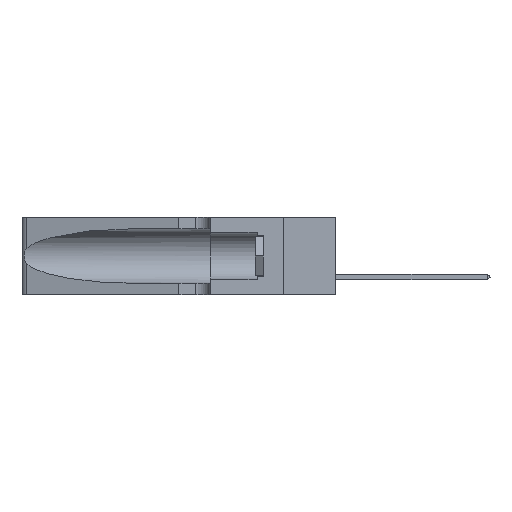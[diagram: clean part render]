
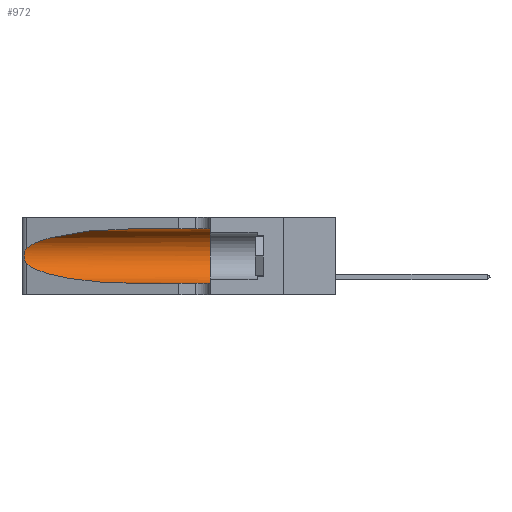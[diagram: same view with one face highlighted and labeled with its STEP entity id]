
A CAD part, left-side view. The second image highlights one B-rep face of the part: STEP entity #972.
In plain terms, the highlighted cylindrical face has radius 3.308 mm (diameter 6.617 mm), a partial arc.
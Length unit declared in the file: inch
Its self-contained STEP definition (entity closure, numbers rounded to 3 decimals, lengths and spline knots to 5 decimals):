
#449 = CARTESIAN_POINT ( 'NONE',  ( 0.25487, 1.22718, 0.14631 ) ) ;
#681 = AXIS2_PLACEMENT_3D ( 'NONE', #48980, #38455, #11279 ) ;
#937 = CARTESIAN_POINT ( 'NONE',  ( 0.25487, 1.22718, 0.22369 ) ) ;
#972 = ADVANCED_FACE ( 'NONE', ( #47488 ), #1754, .F. ) ;
#1268 = ORIENTED_EDGE ( 'NONE', *, *, #25857, .F. ) ;
#1339 = CARTESIAN_POINT ( 'NONE',  ( 0.1305, 1.61858, 0.185 ) ) ;
#1754 = CYLINDRICAL_SURFACE ( 'NONE', #24909, 0.13025 ) ;
#3576 = CARTESIAN_POINT ( 'NONE',  ( 0.2373, 1.15595, 0.08982 ) ) ;
#4775 = CARTESIAN_POINT ( 'NONE',  ( 0.1305, 0.35, 0.05475 ) ) ;
#6134 = CARTESIAN_POINT ( 'NONE',  ( 0.25555, 1.22994, 0.2215 ) ) ;
#6475 = CARTESIAN_POINT ( 'NONE',  ( 0.25787, 1.23484, 0.2124 ) ) ;
#8892 = CARTESIAN_POINT ( 'NONE',  ( 0.1305, 0.72297, 0.05475 ) ) ;
#11030 = CARTESIAN_POINT ( 'NONE',  ( 0.26017, 1.23833, 0.17102 ) ) ;
#11052 = ORIENTED_EDGE ( 'NONE', *, *, #31188, .F. ) ;
#11162 = EDGE_CURVE ( 'NONE', #36340, #18987, #49868, .T. ) ;
#11279 = DIRECTION ( 'NONE',  ( 0., 0., 1. ) ) ;
#11449 = ORIENTED_EDGE ( 'NONE', *, *, #23421, .T. ) ;
#12258 = CARTESIAN_POINT ( 'NONE',  ( 0.25555, 1.22993, 0.14849 ) ) ;
#12418 = CARTESIAN_POINT ( 'NONE',  ( 0.1305, 1.61858, 0.05475 ) ) ;
#14858 = CARTESIAN_POINT ( 'NONE',  ( 0.1305, 0.35, 0.31525 ) ) ;
#15594 = LINE ( 'NONE', #12418, #34826 ) ;
#16298 = DIRECTION ( 'NONE',  ( 0., -1., 0. ) ) ;
#17581 = ORIENTED_EDGE ( 'NONE', *, *, #11162, .T. ) ;
#18987 = VERTEX_POINT ( 'NONE', #34523 ) ;
#19622 = CARTESIAN_POINT ( 'NONE',  ( 0.1305, 0.72297, 0.31525 ) ) ;
#19818 = DIRECTION ( 'NONE',  ( 0., 0., -1. ) ) ;
#20849 = EDGE_CURVE ( 'NONE', #45648, #36340, #28413, .T. ) ;
#20927 = VERTEX_POINT ( 'NONE', #4775 ) ;
#22044 = VERTEX_POINT ( 'NONE', #14858 ) ;
#23013 = CARTESIAN_POINT ( 'NONE',  ( 0.25639, 1.23186, 0.15144 ) ) ;
#23421 = EDGE_CURVE ( 'NONE', #18987, #20927, #15594, .T. ) ;
#24909 = AXIS2_PLACEMENT_3D ( 'NONE', #1339, #16298, #19818 ) ;
#25857 = EDGE_CURVE ( 'NONE', #41160, #22044, #27773, .T. ) ;
#25876 = CARTESIAN_POINT ( 'NONE',  ( 0.25487, 1.22718, 0.14631 ) ) ;
#26415 = CARTESIAN_POINT ( 'NONE',  ( 0.25789, 1.23486, 0.15765 ) ) ;
#27773 = LINE ( 'NONE', #43423, #40519 ) ;
#28056 = DIRECTION ( 'NONE',  ( 0., -1., 0. ) ) ;
#28413 = B_SPLINE_CURVE_WITH_KNOTS ( 'NONE', 3,
 ( #44272, #6134, #45478, #6475, #45305, #33151, #38370, #46120, #11030, #37879, #26415, #23013, #12258, #449 ),
 .UNSPECIFIED., .F., .F.,
 ( 4, 2, 2, 2, 2, 2, 4 ),
 ( 0., 0.00027, 0.00053, 0.00107, 0.0016, 0.00187, 0.00214 ),
 .UNSPECIFIED. ) ;
#29901 = CARTESIAN_POINT ( 'NONE',  ( 0.1305, 0.72297, 0.31525 ) ) ;
#30822 = CIRCLE ( 'NONE', #681, 0.13025 ) ;
#31183 = CARTESIAN_POINT ( 'NONE',  ( 0.18966, 0.96281, 0.31525 ) ) ;
#31188 = EDGE_CURVE ( 'NONE', #22044, #20927, #30822, .T. ) ;
#33151 = CARTESIAN_POINT ( 'NONE',  ( 0.26018, 1.23835, 0.19895 ) ) ;
#34523 = CARTESIAN_POINT ( 'NONE',  ( 0.1305, 0.72297, 0.05475 ) ) ;
#34826 = VECTOR ( 'NONE', #47391, 39.37008 ) ;
#35974 = CARTESIAN_POINT ( 'NONE',  ( 0.18966, 0.96281, 0.05475 ) ) ;
#36340 = VERTEX_POINT ( 'NONE', #42145 ) ;
#37879 = CARTESIAN_POINT ( 'NONE',  ( 0.25856, 1.23593, 0.16098 ) ) ;
#38370 = CARTESIAN_POINT ( 'NONE',  ( 0.26075, 1.23896, 0.19203 ) ) ;
#38455 = DIRECTION ( 'NONE',  ( 0., 1., 0. ) ) ;
#39304 = CARTESIAN_POINT ( 'NONE',  ( 0.2373, 1.15595, 0.28018 ) ) ;
#39447 = EDGE_LOOP ( 'NONE', ( #41276, #40803, #17581, #11449, #11052, #1268 ) ) ;
#40519 = VECTOR ( 'NONE', #28056, 39.37008 ) ;
#40586 = EDGE_CURVE ( 'NONE', #41160, #45648, #46941, .T. ) ;
#40803 = ORIENTED_EDGE ( 'NONE', *, *, #20849, .T. ) ;
#41160 = VERTEX_POINT ( 'NONE', #29901 ) ;
#41276 = ORIENTED_EDGE ( 'NONE', *, *, #40586, .T. ) ;
#42145 = CARTESIAN_POINT ( 'NONE',  ( 0.25487, 1.22718, 0.14631 ) ) ;
#43423 = CARTESIAN_POINT ( 'NONE',  ( 0.1305, 1.61858, 0.31525 ) ) ;
#44272 = CARTESIAN_POINT ( 'NONE',  ( 0.25487, 1.22718, 0.22369 ) ) ;
#45004 = CARTESIAN_POINT ( 'NONE',  ( 0.25487, 1.22718, 0.22369 ) ) ;
#45305 = CARTESIAN_POINT ( 'NONE',  ( 0.25854, 1.2359, 0.20912 ) ) ;
#45478 = CARTESIAN_POINT ( 'NONE',  ( 0.25639, 1.23184, 0.21858 ) ) ;
#45648 = VERTEX_POINT ( 'NONE', #45004 ) ;
#46120 = CARTESIAN_POINT ( 'NONE',  ( 0.26075, 1.23896, 0.178 ) ) ;
#46941 =( BOUNDED_CURVE ( )  B_SPLINE_CURVE ( 3, ( #19622, #31183, #39304, #937 ),
 .UNSPECIFIED., .F., .F. ) 
 B_SPLINE_CURVE_WITH_KNOTS ( ( 4, 4 ),
 ( 1.5708, 2.84003 ),
 .UNSPECIFIED. ) 
 CURVE ( )  GEOMETRIC_REPRESENTATION_ITEM ( )  RATIONAL_B_SPLINE_CURVE ( ( 1., 0.87, 0.87, 1. ) ) 
 REPRESENTATION_ITEM ( '' )  );
#47391 = DIRECTION ( 'NONE',  ( 0., -1., 0. ) ) ;
#47488 = FACE_OUTER_BOUND ( 'NONE', #39447, .T. ) ;
#48980 = CARTESIAN_POINT ( 'NONE',  ( 0.1305, 0.35, 0.185 ) ) ;
#49868 =( BOUNDED_CURVE ( )  B_SPLINE_CURVE ( 3, ( #25876, #3576, #35974, #8892 ),
 .UNSPECIFIED., .F., .F. ) 
 B_SPLINE_CURVE_WITH_KNOTS ( ( 4, 4 ),
 ( 3.44316, 4.71239 ),
 .UNSPECIFIED. ) 
 CURVE ( )  GEOMETRIC_REPRESENTATION_ITEM ( )  RATIONAL_B_SPLINE_CURVE ( ( 1., 0.87, 0.87, 1. ) ) 
 REPRESENTATION_ITEM ( '' )  );
